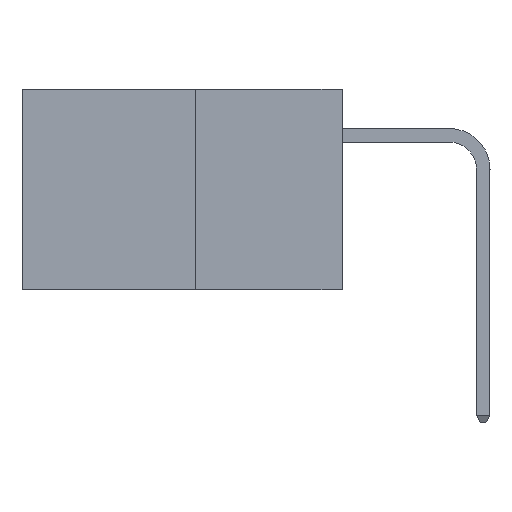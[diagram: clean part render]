
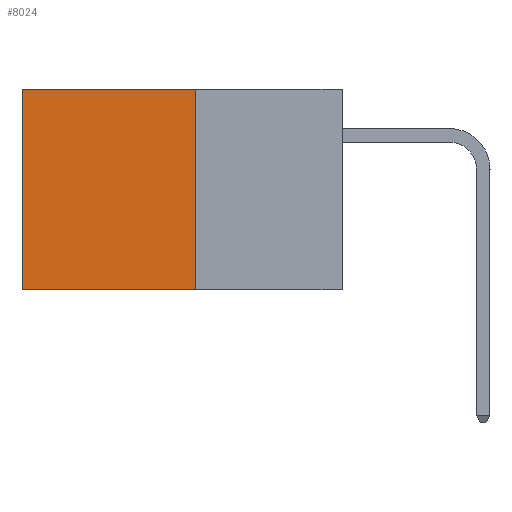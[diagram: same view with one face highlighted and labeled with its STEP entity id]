
A CAD part, left-side view. The second image highlights one B-rep face of the part: STEP entity #8024.
In plain terms, the highlighted planar face has unit normal (-1, 0, 0).
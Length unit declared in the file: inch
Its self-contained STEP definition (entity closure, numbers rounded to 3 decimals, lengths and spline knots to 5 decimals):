
#759 = VECTOR ( 'NONE', #14533, 39.37008 ) ;
#917 = DIRECTION ( 'NONE',  ( 0., 1., 0. ) ) ;
#1239 = ORIENTED_EDGE ( 'NONE', *, *, #2561, .T. ) ;
#1254 = VERTEX_POINT ( 'NONE', #11571 ) ;
#2169 = LINE ( 'NONE', #3915, #8642 ) ;
#2220 = PLANE ( 'NONE',  #12527 ) ;
#2561 = EDGE_CURVE ( 'NONE', #1254, #10092, #10711, .T. ) ;
#3015 = VERTEX_POINT ( 'NONE', #8374 ) ;
#3915 = CARTESIAN_POINT ( 'NONE',  ( 0.277, 0.27, 0. ) ) ;
#4250 = CARTESIAN_POINT ( 'NONE',  ( 0.277, 0.27, 0. ) ) ;
#4868 = DIRECTION ( 'NONE',  ( 1., 0., 0. ) ) ;
#5145 = EDGE_CURVE ( 'NONE', #6346, #3015, #7849, .T. ) ;
#5154 = EDGE_LOOP ( 'NONE', ( #1239, #8054, #15350, #7197 ) ) ;
#6346 = VERTEX_POINT ( 'NONE', #4250 ) ;
#7197 = ORIENTED_EDGE ( 'NONE', *, *, #13326, .T. ) ;
#7311 = CARTESIAN_POINT ( 'NONE',  ( 0.277, 0.27, -0.37 ) ) ;
#7457 = VECTOR ( 'NONE', #9732, 39.37008 ) ;
#7764 = DIRECTION ( 'NONE',  ( 0., 1., 0. ) ) ;
#7840 = LINE ( 'NONE', #16128, #10429 ) ;
#7849 = LINE ( 'NONE', #7311, #7457 ) ;
#8024 = ADVANCED_FACE ( 'NONE', ( #16425 ), #2220, .F. ) ;
#8054 = ORIENTED_EDGE ( 'NONE', *, *, #10649, .F. ) ;
#8374 = CARTESIAN_POINT ( 'NONE',  ( 0.277, 0.27, -0.37 ) ) ;
#8642 = VECTOR ( 'NONE', #7764, 39.37008 ) ;
#9674 = CARTESIAN_POINT ( 'NONE',  ( 0.277, 0.59, -0.37 ) ) ;
#9732 = DIRECTION ( 'NONE',  ( 0., 0., -1. ) ) ;
#10092 = VERTEX_POINT ( 'NONE', #10251 ) ;
#10251 = CARTESIAN_POINT ( 'NONE',  ( 0.277, 0.59, -0.37 ) ) ;
#10429 = VECTOR ( 'NONE', #917, 39.37008 ) ;
#10649 = EDGE_CURVE ( 'NONE', #3015, #10092, #7840, .T. ) ;
#10711 = LINE ( 'NONE', #9674, #759 ) ;
#11571 = CARTESIAN_POINT ( 'NONE',  ( 0.277, 0.59, 0. ) ) ;
#12438 = CARTESIAN_POINT ( 'NONE',  ( 0.277, 0.27, -0.37 ) ) ;
#12527 = AXIS2_PLACEMENT_3D ( 'NONE', #12438, #4868, #13666 ) ;
#13326 = EDGE_CURVE ( 'NONE', #6346, #1254, #2169, .T. ) ;
#13666 = DIRECTION ( 'NONE',  ( 0., 0., -1. ) ) ;
#14533 = DIRECTION ( 'NONE',  ( 0., 0., -1. ) ) ;
#15350 = ORIENTED_EDGE ( 'NONE', *, *, #5145, .F. ) ;
#16128 = CARTESIAN_POINT ( 'NONE',  ( 0.277, 0.27, -0.37 ) ) ;
#16425 = FACE_OUTER_BOUND ( 'NONE', #5154, .T. ) ;
